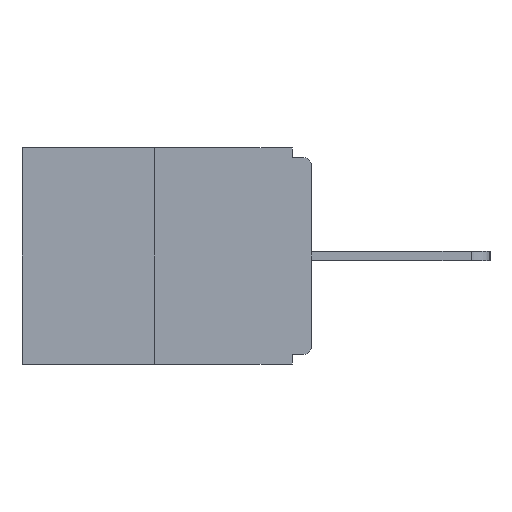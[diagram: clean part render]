
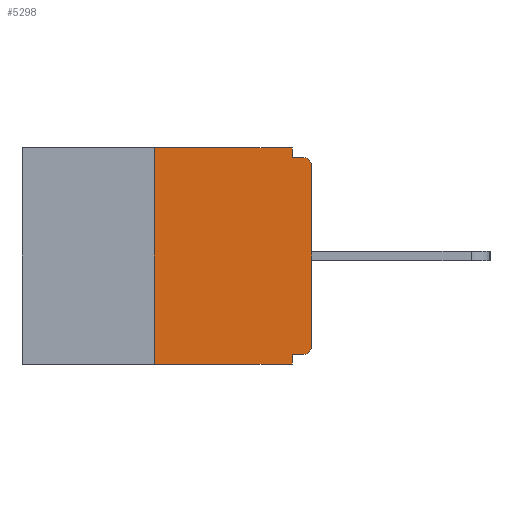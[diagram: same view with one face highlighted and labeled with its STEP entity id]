
A CAD part, left-side view. The second image highlights one B-rep face of the part: STEP entity #5298.
In plain terms, the highlighted planar face has unit normal (-1, 0, 0).
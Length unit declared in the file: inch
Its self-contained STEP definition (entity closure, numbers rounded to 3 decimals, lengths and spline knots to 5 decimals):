
#204 = LINE ( 'NONE', #9441, #9542 ) ;
#334 = EDGE_CURVE ( 'NONE', #8478, #7138, #6320, .T. ) ;
#347 = LINE ( 'NONE', #14980, #6120 ) ;
#438 = EDGE_CURVE ( 'NONE', #10434, #10351, #347, .T. ) ;
#476 = EDGE_CURVE ( 'NONE', #1189, #2106, #12507, .T. ) ;
#501 = EDGE_CURVE ( 'NONE', #8478, #10351, #8153, .T. ) ;
#967 = DIRECTION ( 'NONE',  ( 0., 1., 0. ) ) ;
#989 = CARTESIAN_POINT ( 'NONE',  ( 0., 0.46, 0. ) ) ;
#1189 = VERTEX_POINT ( 'NONE', #2236 ) ;
#1279 = ORIENTED_EDGE ( 'NONE', *, *, #15312, .T. ) ;
#1694 = CARTESIAN_POINT ( 'NONE',  ( 0., 0.46, 0. ) ) ;
#2106 = VERTEX_POINT ( 'NONE', #4140 ) ;
#2145 = VECTOR ( 'NONE', #11628, 39.37008 ) ;
#2236 = CARTESIAN_POINT ( 'NONE',  ( 0., 0.031, 0. ) ) ;
#2877 = VERTEX_POINT ( 'NONE', #6756 ) ;
#3248 = DIRECTION ( 'NONE',  ( 0., -1., 0. ) ) ;
#3756 = CARTESIAN_POINT ( 'NONE',  ( 0., 0.015, -0.03 ) ) ;
#3932 = EDGE_CURVE ( 'NONE', #2877, #7653, #12811, .T. ) ;
#3967 = CARTESIAN_POINT ( 'NONE',  ( 0., 0.031, 0. ) ) ;
#4140 = CARTESIAN_POINT ( 'NONE',  ( 0., 0.031, -0.015 ) ) ;
#4386 = CARTESIAN_POINT ( 'NONE',  ( 0., 0.25, -0.343 ) ) ;
#4910 = ORIENTED_EDGE ( 'NONE', *, *, #3932, .T. ) ;
#4921 = EDGE_LOOP ( 'NONE', ( #5280, #5655, #13163, #6958, #10546, #13733, #1279, #4910, #8442, #12069 ) ) ;
#4995 = CARTESIAN_POINT ( 'NONE',  ( 0., 0., -0.313 ) ) ;
#5117 = CARTESIAN_POINT ( 'NONE',  ( 0., 0., -0.015 ) ) ;
#5280 = ORIENTED_EDGE ( 'NONE', *, *, #5669, .F. ) ;
#5298 = ADVANCED_FACE ( 'NONE', ( #7500 ), #10839, .F. ) ;
#5305 = CARTESIAN_POINT ( 'NONE',  ( 0., 0.015, -0.313 ) ) ;
#5308 = DIRECTION ( 'NONE',  ( -1., 0., 0. ) ) ;
#5642 = LINE ( 'NONE', #5117, #6009 ) ;
#5655 = ORIENTED_EDGE ( 'NONE', *, *, #334, .F. ) ;
#5669 = EDGE_CURVE ( 'NONE', #7138, #1189, #11483, .T. ) ;
#5810 = VECTOR ( 'NONE', #8088, 39.37008 ) ;
#6009 = VECTOR ( 'NONE', #12318, 39.37008 ) ;
#6120 = VECTOR ( 'NONE', #14483, 39.37008 ) ;
#6320 = LINE ( 'NONE', #12587, #8711 ) ;
#6595 = EDGE_CURVE ( 'NONE', #7488, #11704, #8190, .T. ) ;
#6756 = CARTESIAN_POINT ( 'NONE',  ( 0., 0., -0.03 ) ) ;
#6958 = ORIENTED_EDGE ( 'NONE', *, *, #438, .F. ) ;
#7023 = CARTESIAN_POINT ( 'NONE',  ( 0., 0.015, -0.328 ) ) ;
#7138 = VERTEX_POINT ( 'NONE', #13670 ) ;
#7488 = VERTEX_POINT ( 'NONE', #7023 ) ;
#7500 = FACE_OUTER_BOUND ( 'NONE', #4921, .T. ) ;
#7653 = VERTEX_POINT ( 'NONE', #12250 ) ;
#7777 = VECTOR ( 'NONE', #3248, 39.37008 ) ;
#7846 = VECTOR ( 'NONE', #11053, 39.37008 ) ;
#8088 = DIRECTION ( 'NONE',  ( 0., 0., 1. ) ) ;
#8153 = LINE ( 'NONE', #12103, #7777 ) ;
#8190 = CIRCLE ( 'NONE', #8308, 0.015 ) ;
#8308 = AXIS2_PLACEMENT_3D ( 'NONE', #5305, #5308, #9060 ) ;
#8442 = ORIENTED_EDGE ( 'NONE', *, *, #8870, .F. ) ;
#8478 = VERTEX_POINT ( 'NONE', #4386 ) ;
#8610 = CARTESIAN_POINT ( 'NONE',  ( 0., 0.031, -0.328 ) ) ;
#8647 = DIRECTION ( 'NONE',  ( 0., 0., -1. ) ) ;
#8711 = VECTOR ( 'NONE', #10816, 39.37008 ) ;
#8870 = EDGE_CURVE ( 'NONE', #2106, #7653, #5642, .T. ) ;
#9060 = DIRECTION ( 'NONE',  ( 0., 0., -1. ) ) ;
#9294 = EDGE_CURVE ( 'NONE', #7488, #10434, #204, .T. ) ;
#9441 = CARTESIAN_POINT ( 'NONE',  ( 0., 0., -0.328 ) ) ;
#9542 = VECTOR ( 'NONE', #967, 39.37008 ) ;
#10351 = VERTEX_POINT ( 'NONE', #10999 ) ;
#10434 = VERTEX_POINT ( 'NONE', #8610 ) ;
#10546 = ORIENTED_EDGE ( 'NONE', *, *, #9294, .F. ) ;
#10816 = DIRECTION ( 'NONE',  ( 0., 0., 1. ) ) ;
#10839 = PLANE ( 'NONE',  #14643 ) ;
#10999 = CARTESIAN_POINT ( 'NONE',  ( 0., 0.031, -0.343 ) ) ;
#11053 = DIRECTION ( 'NONE',  ( 0., -1., 0. ) ) ;
#11483 = LINE ( 'NONE', #989, #7846 ) ;
#11628 = DIRECTION ( 'NONE',  ( 0., 0., -1. ) ) ;
#11704 = VERTEX_POINT ( 'NONE', #4995 ) ;
#12069 = ORIENTED_EDGE ( 'NONE', *, *, #476, .F. ) ;
#12103 = CARTESIAN_POINT ( 'NONE',  ( 0., 0.46, -0.343 ) ) ;
#12250 = CARTESIAN_POINT ( 'NONE',  ( 0., 0.015, -0.015 ) ) ;
#12318 = DIRECTION ( 'NONE',  ( 0., -1., 0. ) ) ;
#12451 = DIRECTION ( 'NONE',  ( -1., 0., 0. ) ) ;
#12507 = LINE ( 'NONE', #3967, #2145 ) ;
#12587 = CARTESIAN_POINT ( 'NONE',  ( 0., 0.25, 0. ) ) ;
#12811 = CIRCLE ( 'NONE', #12938, 0.015 ) ;
#12938 = AXIS2_PLACEMENT_3D ( 'NONE', #3756, #12451, #13712 ) ;
#13163 = ORIENTED_EDGE ( 'NONE', *, *, #501, .T. ) ;
#13670 = CARTESIAN_POINT ( 'NONE',  ( 0., 0.25, 0. ) ) ;
#13712 = DIRECTION ( 'NONE',  ( 0., 0., -1. ) ) ;
#13733 = ORIENTED_EDGE ( 'NONE', *, *, #6595, .T. ) ;
#14335 = DIRECTION ( 'NONE',  ( 1., 0., 0. ) ) ;
#14483 = DIRECTION ( 'NONE',  ( 0., 0., -1. ) ) ;
#14603 = LINE ( 'NONE', #15272, #5810 ) ;
#14643 = AXIS2_PLACEMENT_3D ( 'NONE', #1694, #14335, #8647 ) ;
#14980 = CARTESIAN_POINT ( 'NONE',  ( 0., 0.031, -0.343 ) ) ;
#15272 = CARTESIAN_POINT ( 'NONE',  ( 0., 0., 0. ) ) ;
#15312 = EDGE_CURVE ( 'NONE', #11704, #2877, #14603, .T. ) ;
